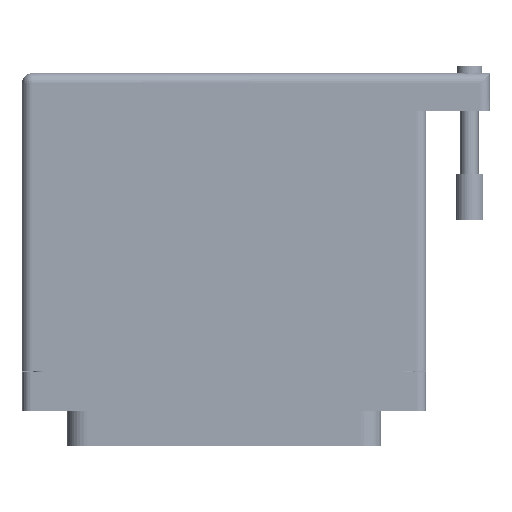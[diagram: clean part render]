
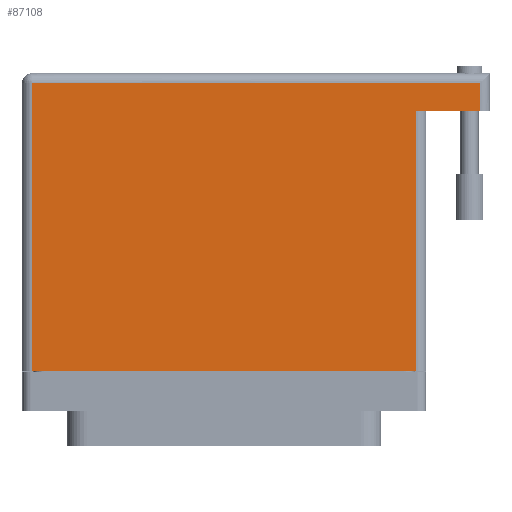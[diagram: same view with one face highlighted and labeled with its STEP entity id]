
A CAD part, front view. The second image highlights one B-rep face of the part: STEP entity #87108.
In plain terms, the highlighted face is planar.
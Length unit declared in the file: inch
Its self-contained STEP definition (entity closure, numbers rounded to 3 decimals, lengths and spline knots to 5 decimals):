
#2036 = EDGE_CURVE ( 'NONE', #24396, #48933, #38721, .T. ) ;
#3081 = EDGE_LOOP ( 'NONE', ( #4025, #23962, #41035, #33049, #80671, #64963 ) ) ;
#3689 = VECTOR ( 'NONE', #18943, 39.37008 ) ;
#4025 = ORIENTED_EDGE ( 'NONE', *, *, #17791, .T. ) ;
#4821 = CARTESIAN_POINT ( 'NONE',  ( -1.3075, 1.86, 0.765 ) ) ;
#5865 = LINE ( 'NONE', #25281, #3689 ) ;
#7952 = VECTOR ( 'NONE', #74130, 39.37008 ) ;
#10976 = CARTESIAN_POINT ( 'NONE',  ( -1.3775, 1.86, 0.765 ) ) ;
#13609 = EDGE_CURVE ( 'NONE', #26063, #48933, #53398, .T. ) ;
#15687 = VERTEX_POINT ( 'NONE', #55667 ) ;
#17791 = EDGE_CURVE ( 'NONE', #74967, #24396, #5865, .T. ) ;
#18563 = DIRECTION ( 'NONE',  ( -1., 0., 0. ) ) ;
#18943 = DIRECTION ( 'NONE',  ( 1., 0., 0. ) ) ;
#21146 = VECTOR ( 'NONE', #25426, 39.37008 ) ;
#22875 = CARTESIAN_POINT ( 'NONE',  ( -1.3075, -0.1, 0.765 ) ) ;
#23962 = ORIENTED_EDGE ( 'NONE', *, *, #2036, .T. ) ;
#24396 = VERTEX_POINT ( 'NONE', #59456 ) ;
#24677 = CARTESIAN_POINT ( 'NONE',  ( -1.3075, -0.1, 0.765 ) ) ;
#24958 = LINE ( 'NONE', #10976, #7952 ) ;
#25281 = CARTESIAN_POINT ( 'NONE',  ( -1.3775, -0.1, 0.765 ) ) ;
#25426 = DIRECTION ( 'NONE',  ( -1., 0., 0. ) ) ;
#26063 = VERTEX_POINT ( 'NONE', #79680 ) ;
#31220 = FACE_OUTER_BOUND ( 'NONE', #3081, .T. ) ;
#33049 = ORIENTED_EDGE ( 'NONE', *, *, #74207, .T. ) ;
#33153 = EDGE_CURVE ( 'NONE', #15687, #56837, #24958, .T. ) ;
#38721 = LINE ( 'NONE', #66697, #51107 ) ;
#39569 = VECTOR ( 'NONE', #85562, 39.37008 ) ;
#41035 = ORIENTED_EDGE ( 'NONE', *, *, #13609, .F. ) ;
#42388 = VECTOR ( 'NONE', #83955, 39.37008 ) ;
#45237 = CARTESIAN_POINT ( 'NONE',  ( 1.3075, 1.674, 0.765 ) ) ;
#45663 = PLANE ( 'NONE',  #83277 ) ;
#46816 = EDGE_CURVE ( 'NONE', #56837, #74967, #58047, .T. ) ;
#47885 = LINE ( 'NONE', #68629, #42388 ) ;
#48933 = VERTEX_POINT ( 'NONE', #45237 ) ;
#51107 = VECTOR ( 'NONE', #66233, 39.37008 ) ;
#53398 = LINE ( 'NONE', #74144, #21146 ) ;
#55667 = CARTESIAN_POINT ( 'NONE',  ( 1.7425, 1.86, 0.765 ) ) ;
#56837 = VERTEX_POINT ( 'NONE', #4821 ) ;
#58047 = LINE ( 'NONE', #22875, #39569 ) ;
#59456 = CARTESIAN_POINT ( 'NONE',  ( 1.3075, -0.1, 0.765 ) ) ;
#64963 = ORIENTED_EDGE ( 'NONE', *, *, #46816, .T. ) ;
#65494 = CARTESIAN_POINT ( 'NONE',  ( -1.3775, 1.93, 0.765 ) ) ;
#66233 = DIRECTION ( 'NONE',  ( 0., 1., 0. ) ) ;
#66697 = CARTESIAN_POINT ( 'NONE',  ( 1.3075, 1.674, 0.765 ) ) ;
#68629 = CARTESIAN_POINT ( 'NONE',  ( 1.7425, 1.93, 0.765 ) ) ;
#74130 = DIRECTION ( 'NONE',  ( -1., 0., 0. ) ) ;
#74144 = CARTESIAN_POINT ( 'NONE',  ( 1.8125, 1.674, 0.765 ) ) ;
#74207 = EDGE_CURVE ( 'NONE', #26063, #15687, #47885, .T. ) ;
#74967 = VERTEX_POINT ( 'NONE', #24677 ) ;
#79680 = CARTESIAN_POINT ( 'NONE',  ( 1.7425, 1.674, 0.765 ) ) ;
#80671 = ORIENTED_EDGE ( 'NONE', *, *, #33153, .T. ) ;
#83277 = AXIS2_PLACEMENT_3D ( 'NONE', #65494, #86251, #18563 ) ;
#83955 = DIRECTION ( 'NONE',  ( 0., 1., 0. ) ) ;
#85562 = DIRECTION ( 'NONE',  ( 0., -1., 0. ) ) ;
#86251 = DIRECTION ( 'NONE',  ( 0., 0., -1. ) ) ;
#87108 = ADVANCED_FACE ( 'NONE', ( #31220 ), #45663, .F. ) ;
